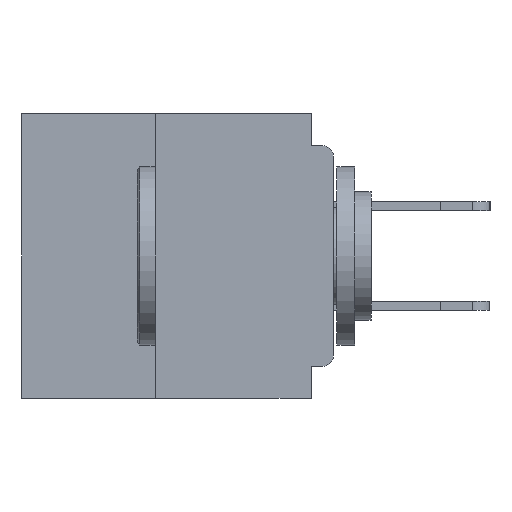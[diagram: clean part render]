
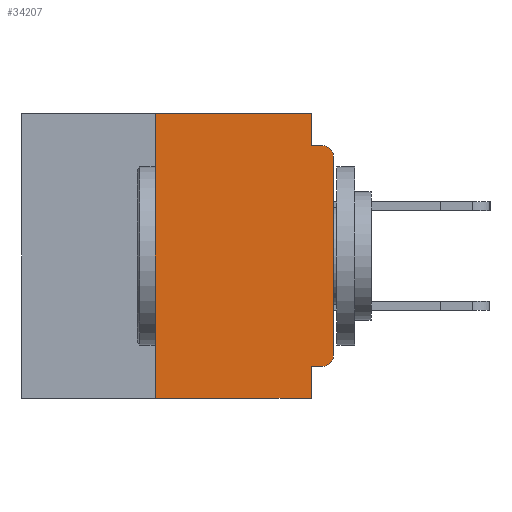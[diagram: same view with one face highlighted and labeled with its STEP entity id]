
A CAD part, left-side view. The second image highlights one B-rep face of the part: STEP entity #34207.
In plain terms, the highlighted planar face has unit normal (-1, 0, 0).
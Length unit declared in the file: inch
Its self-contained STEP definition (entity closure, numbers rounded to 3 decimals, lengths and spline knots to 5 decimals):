
#233 = EDGE_CURVE ( 'NONE', #38420, #16008, #35742, .T. ) ;
#799 = DIRECTION ( 'NONE',  ( 0., -1., 0. ) ) ;
#1569 = AXIS2_PLACEMENT_3D ( 'NONE', #31086, #7986, #34970 ) ;
#1625 = VERTEX_POINT ( 'NONE', #33051 ) ;
#1808 = ORIENTED_EDGE ( 'NONE', *, *, #28080, .F. ) ;
#3030 = DIRECTION ( 'NONE',  ( 0., 1., 0. ) ) ;
#4231 = VECTOR ( 'NONE', #46455, 39.37008 ) ;
#5168 = CARTESIAN_POINT ( 'NONE',  ( 0., 0.015, -0.045 ) ) ;
#5903 = VECTOR ( 'NONE', #12216, 39.37008 ) ;
#5982 = ORIENTED_EDGE ( 'NONE', *, *, #38416, .F. ) ;
#6188 = LINE ( 'NONE', #48993, #35766 ) ;
#6546 = CARTESIAN_POINT ( 'NONE',  ( 0., 0.031, -0.4 ) ) ;
#6609 = ORIENTED_EDGE ( 'NONE', *, *, #47066, .F. ) ;
#7811 = ORIENTED_EDGE ( 'NONE', *, *, #26541, .T. ) ;
#7880 = CARTESIAN_POINT ( 'NONE',  ( 0., 0.25, -0.4 ) ) ;
#7986 = DIRECTION ( 'NONE',  ( -1., 0., 0. ) ) ;
#9074 = VECTOR ( 'NONE', #15359, 39.37008 ) ;
#10665 = CARTESIAN_POINT ( 'NONE',  ( 0., 0.031, -0.4 ) ) ;
#11204 = VERTEX_POINT ( 'NONE', #10665 ) ;
#11492 = CARTESIAN_POINT ( 'NONE',  ( 0., 0., -0.34 ) ) ;
#11710 = CARTESIAN_POINT ( 'NONE',  ( 0., 0.015, -0.34 ) ) ;
#12216 = DIRECTION ( 'NONE',  ( 0., -1., 0. ) ) ;
#13676 = VERTEX_POINT ( 'NONE', #18186 ) ;
#14201 = DIRECTION ( 'NONE',  ( 0., -1., 0. ) ) ;
#14800 = VERTEX_POINT ( 'NONE', #40251 ) ;
#15359 = DIRECTION ( 'NONE',  ( 0., 0., -1. ) ) ;
#15575 = ORIENTED_EDGE ( 'NONE', *, *, #46119, .T. ) ;
#15594 = DIRECTION ( 'NONE',  ( 0., 0., -1. ) ) ;
#15603 = DIRECTION ( 'NONE',  ( 0., 0., 1. ) ) ;
#16008 = VERTEX_POINT ( 'NONE', #35927 ) ;
#16875 = VECTOR ( 'NONE', #15603, 39.37008 ) ;
#17001 = VECTOR ( 'NONE', #799, 39.37008 ) ;
#17830 = CIRCLE ( 'NONE', #22272, 0.015 ) ;
#18186 = CARTESIAN_POINT ( 'NONE',  ( 0., 0.031, -0.355 ) ) ;
#18893 = EDGE_LOOP ( 'NONE', ( #15575, #19188, #35137, #34328, #25294, #5982, #19832, #1808, #6609, #7811 ) ) ;
#18897 = CARTESIAN_POINT ( 'NONE',  ( 0., 0.437, 0. ) ) ;
#19188 = ORIENTED_EDGE ( 'NONE', *, *, #34280, .T. ) ;
#19461 = CARTESIAN_POINT ( 'NONE',  ( 0., 0.25, 0. ) ) ;
#19832 = ORIENTED_EDGE ( 'NONE', *, *, #33249, .T. ) ;
#20243 = CIRCLE ( 'NONE', #1569, 0.015 ) ;
#22272 = AXIS2_PLACEMENT_3D ( 'NONE', #11710, #38755, #15594 ) ;
#22650 = VERTEX_POINT ( 'NONE', #48650 ) ;
#22806 = DIRECTION ( 'NONE',  ( 0., 0., -1. ) ) ;
#22966 = EDGE_CURVE ( 'NONE', #43640, #30524, #46467, .T. ) ;
#23891 = FACE_OUTER_BOUND ( 'NONE', #18893, .T. ) ;
#25294 = ORIENTED_EDGE ( 'NONE', *, *, #233, .F. ) ;
#25488 = PLANE ( 'NONE',  #43808 ) ;
#26541 = EDGE_CURVE ( 'NONE', #22650, #30916, #17830, .T. ) ;
#28054 = VECTOR ( 'NONE', #33539, 39.37008 ) ;
#28080 = EDGE_CURVE ( 'NONE', #13676, #11204, #38304, .T. ) ;
#28384 = LINE ( 'NONE', #38518, #9074 ) ;
#28386 = LINE ( 'NONE', #7880, #16875 ) ;
#30524 = VERTEX_POINT ( 'NONE', #5168 ) ;
#30916 = VERTEX_POINT ( 'NONE', #11492 ) ;
#31086 = CARTESIAN_POINT ( 'NONE',  ( 0., 0.015, -0.06 ) ) ;
#33051 = CARTESIAN_POINT ( 'NONE',  ( 0., 0., -0.06 ) ) ;
#33249 = EDGE_CURVE ( 'NONE', #14800, #11204, #45604, .T. ) ;
#33539 = DIRECTION ( 'NONE',  ( 0., 0., -1. ) ) ;
#34207 = ADVANCED_FACE ( 'NONE', ( #23891 ), #25488, .F. ) ;
#34280 = EDGE_CURVE ( 'NONE', #1625, #30524, #20243, .T. ) ;
#34328 = ORIENTED_EDGE ( 'NONE', *, *, #46032, .F. ) ;
#34343 = CARTESIAN_POINT ( 'NONE',  ( 0., 0.031, -0.045 ) ) ;
#34970 = DIRECTION ( 'NONE',  ( 0., 0., -1. ) ) ;
#35136 = CARTESIAN_POINT ( 'NONE',  ( 0., 0., 0. ) ) ;
#35137 = ORIENTED_EDGE ( 'NONE', *, *, #22966, .F. ) ;
#35344 = CARTESIAN_POINT ( 'NONE',  ( 0., 0., -0.045 ) ) ;
#35742 = LINE ( 'NONE', #36301, #42319 ) ;
#35766 = VECTOR ( 'NONE', #3030, 39.37008 ) ;
#35927 = CARTESIAN_POINT ( 'NONE',  ( 0., 0.031, 0. ) ) ;
#36208 = LINE ( 'NONE', #35136, #4231 ) ;
#36301 = CARTESIAN_POINT ( 'NONE',  ( 0., 0.437, 0. ) ) ;
#38304 = LINE ( 'NONE', #6546, #28054 ) ;
#38416 = EDGE_CURVE ( 'NONE', #14800, #38420, #28386, .T. ) ;
#38420 = VERTEX_POINT ( 'NONE', #19461 ) ;
#38518 = CARTESIAN_POINT ( 'NONE',  ( 0., 0.031, 0. ) ) ;
#38755 = DIRECTION ( 'NONE',  ( -1., 0., 0. ) ) ;
#40251 = CARTESIAN_POINT ( 'NONE',  ( 0., 0.25, -0.4 ) ) ;
#42319 = VECTOR ( 'NONE', #14201, 39.37008 ) ;
#43640 = VERTEX_POINT ( 'NONE', #34343 ) ;
#43808 = AXIS2_PLACEMENT_3D ( 'NONE', #18897, #45807, #22806 ) ;
#45604 = LINE ( 'NONE', #46668, #5903 ) ;
#45807 = DIRECTION ( 'NONE',  ( 1., 0., 0. ) ) ;
#46032 = EDGE_CURVE ( 'NONE', #16008, #43640, #28384, .T. ) ;
#46119 = EDGE_CURVE ( 'NONE', #30916, #1625, #36208, .T. ) ;
#46455 = DIRECTION ( 'NONE',  ( 0., 0., 1. ) ) ;
#46467 = LINE ( 'NONE', #35344, #17001 ) ;
#46668 = CARTESIAN_POINT ( 'NONE',  ( 0., 0.437, -0.4 ) ) ;
#47066 = EDGE_CURVE ( 'NONE', #22650, #13676, #6188, .T. ) ;
#48650 = CARTESIAN_POINT ( 'NONE',  ( 0., 0.015, -0.355 ) ) ;
#48993 = CARTESIAN_POINT ( 'NONE',  ( 0., 0., -0.355 ) ) ;
